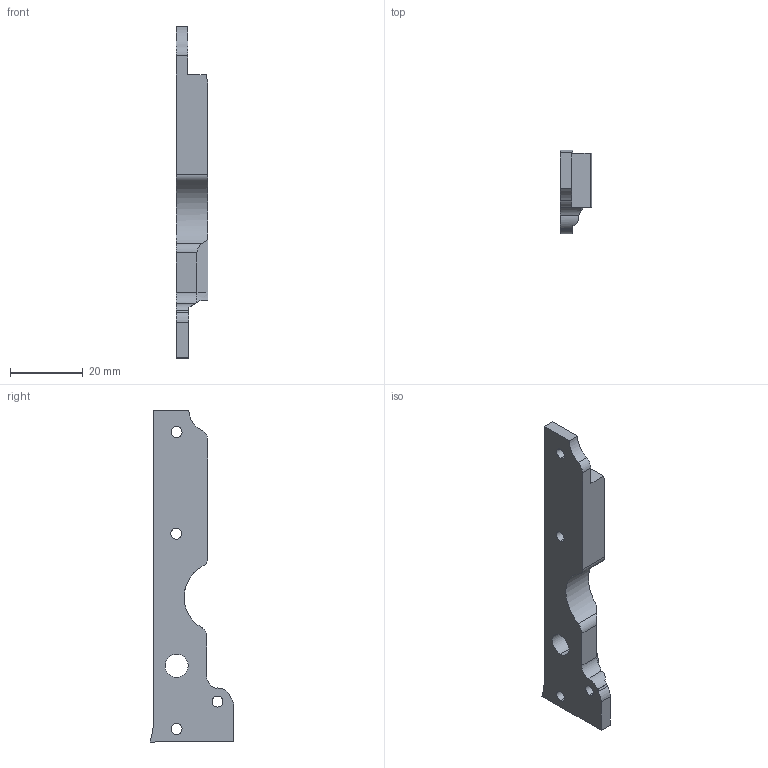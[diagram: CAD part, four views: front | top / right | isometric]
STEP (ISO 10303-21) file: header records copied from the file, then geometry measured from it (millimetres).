
FILE_DESCRIPTION (( 'STEP AP214' ), '1' );
FILE_NAME ('Thunderbolt_Buffer Tower_Split_Arm_Left.STEP', '2021-09-12T03:43:47', ( '' ), ( '' ), 'SwSTEP 2.0', 'SolidWorks 2020', '' );
FILE_SCHEMA (( 'AUTOMOTIVE_DESIGN' ));
Length unit declared in the file: millimetre
Products named in the file (1): Thunderbolt_Buffer Tower_Split_Arm_Left
Bounding box: 8.75 x 23.11 x 91.33 mm (x, y, z)
Volume: 8560.6 mm3; surface area: 4536.4 mm2
Topology: 1 solids, 1 shells, 40 faces, 110 edges, 73 vertices
Faces by surface type: cylinder 22, plane 17, cone 1
Entity records: 1348 total; most frequent: CARTESIAN_POINT 244, DIRECTION 230, ORIENTED_EDGE 220, EDGE_CURVE 110, AXIS2_PLACEMENT_3D 85, VERTEX_POINT 73, LINE 60, VECTOR 60
